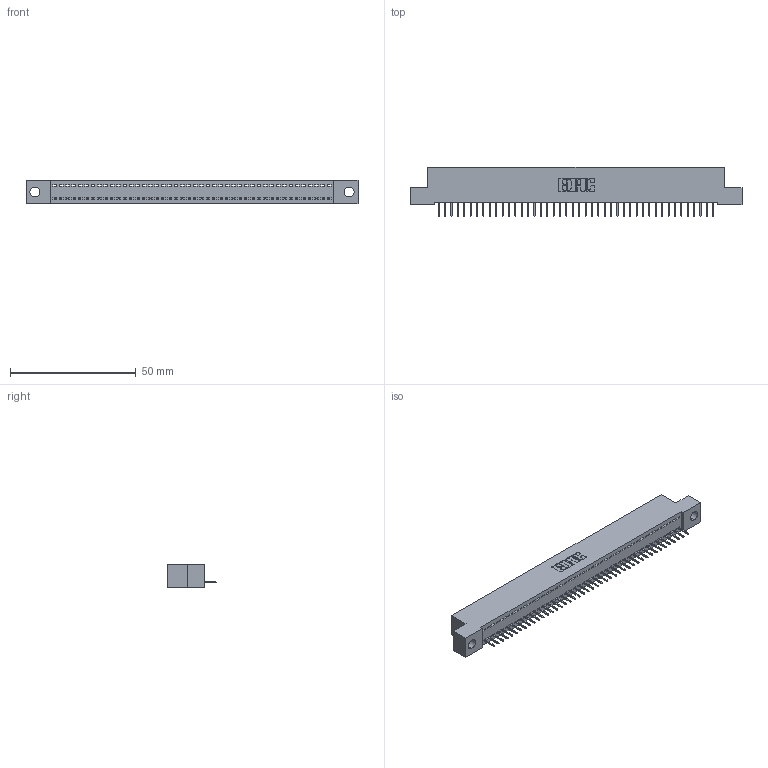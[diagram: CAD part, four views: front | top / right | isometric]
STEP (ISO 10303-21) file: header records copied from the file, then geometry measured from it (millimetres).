
FILE_DESCRIPTION (( 'STEP AP203' ), '1' );
FILE_NAME ('342-044-524-104.STEP', '2019-10-02T19:05:26', ( '' ), ( '' ), 'SwSTEP 2.0', 'SolidWorks 2016', '' );
FILE_SCHEMA (( 'CONFIG_CONTROL_DESIGN' ));
Length unit declared in the file: inch
Products named in the file (3): 342 Part_.156 TH; 345-292-001_345-293-124; 342-044-524-104
Assembly tree (45 placements, depth 2):
  342-044-524-104
    342 Part_.156 TH
    345-292-001_345-293-124  x44
Bounding box: 132.08 x 19.69 x 9.4 mm (x, y, z)
Volume: 11327.3 mm3; surface area: 15949.9 mm2
Topology: 45 solids, 45 shells, 2838 faces, 8219 edges, 5302 vertices
Faces by surface type: plane 2178, cylinder 660
Entity records: 26585 total; most frequent: CARTESIAN_POINT 4590, ORIENTED_EDGE 4570, DIRECTION 3869, EDGE_CURVE 2285, LINE 2161, VECTOR 2161, VERTEX_POINT 1518, AXIS2_PLACEMENT_3D 854
